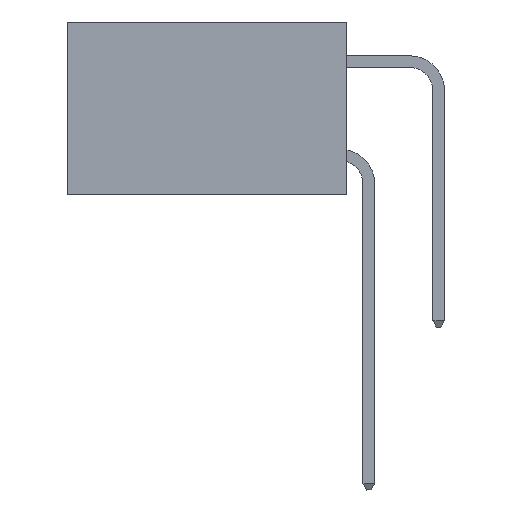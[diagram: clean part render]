
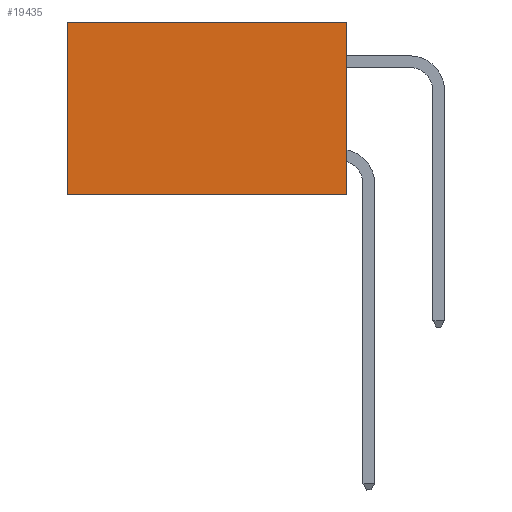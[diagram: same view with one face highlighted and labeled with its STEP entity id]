
A CAD part, left-side view. The second image highlights one B-rep face of the part: STEP entity #19435.
In plain terms, the highlighted planar face has unit normal (-1, 0, 0).
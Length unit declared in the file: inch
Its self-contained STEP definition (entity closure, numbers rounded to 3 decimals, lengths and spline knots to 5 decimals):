
#243 = LINE ( 'NONE', #17175, #26312 ) ;
#957 = AXIS2_PLACEMENT_3D ( 'NONE', #39914, #5919, #27849 ) ;
#1458 = VECTOR ( 'NONE', #9492, 39.37008 ) ;
#1573 = VECTOR ( 'NONE', #36680, 39.37008 ) ;
#1642 = LINE ( 'NONE', #4862, #25771 ) ;
#1814 = EDGE_LOOP ( 'NONE', ( #34650, #26190, #13376, #20717 ) ) ;
#2753 = PLANE ( 'NONE',  #957 ) ;
#4862 = CARTESIAN_POINT ( 'NONE',  ( 0.2875, 0., 0. ) ) ;
#5919 = DIRECTION ( 'NONE',  ( 1., 0., 0. ) ) ;
#8078 = VERTEX_POINT ( 'NONE', #25210 ) ;
#8961 = LINE ( 'NONE', #12013, #1573 ) ;
#9492 = DIRECTION ( 'NONE',  ( 0., 1., 0. ) ) ;
#10827 = LINE ( 'NONE', #34207, #1458 ) ;
#12013 = CARTESIAN_POINT ( 'NONE',  ( 0.2875, 0.6, 0. ) ) ;
#12804 = FACE_OUTER_BOUND ( 'NONE', #1814, .T. ) ;
#13376 = ORIENTED_EDGE ( 'NONE', *, *, #16634, .F. ) ;
#14278 = CARTESIAN_POINT ( 'NONE',  ( 0.2875, 0.6, -0.37 ) ) ;
#16634 = EDGE_CURVE ( 'NONE', #8078, #30290, #243, .T. ) ;
#17175 = CARTESIAN_POINT ( 'NONE',  ( 0.2875, 0., 0. ) ) ;
#17509 = DIRECTION ( 'NONE',  ( 0., 1., 0. ) ) ;
#17941 = VERTEX_POINT ( 'NONE', #14278 ) ;
#19435 = ADVANCED_FACE ( 'NONE', ( #12804 ), #2753, .F. ) ;
#19500 = EDGE_CURVE ( 'NONE', #30290, #17941, #10827, .T. ) ;
#20717 = ORIENTED_EDGE ( 'NONE', *, *, #23862, .T. ) ;
#21933 = CARTESIAN_POINT ( 'NONE',  ( 0.2875, 0., -0.37 ) ) ;
#23862 = EDGE_CURVE ( 'NONE', #8078, #25653, #1642, .T. ) ;
#25210 = CARTESIAN_POINT ( 'NONE',  ( 0.2875, 0., 0. ) ) ;
#25431 = EDGE_CURVE ( 'NONE', #25653, #17941, #8961, .T. ) ;
#25653 = VERTEX_POINT ( 'NONE', #37710 ) ;
#25771 = VECTOR ( 'NONE', #17509, 39.37008 ) ;
#26190 = ORIENTED_EDGE ( 'NONE', *, *, #19500, .F. ) ;
#26312 = VECTOR ( 'NONE', #38700, 39.37008 ) ;
#27849 = DIRECTION ( 'NONE',  ( 0., 0., -1. ) ) ;
#30290 = VERTEX_POINT ( 'NONE', #21933 ) ;
#34207 = CARTESIAN_POINT ( 'NONE',  ( 0.2875, 0., -0.37 ) ) ;
#34650 = ORIENTED_EDGE ( 'NONE', *, *, #25431, .T. ) ;
#36680 = DIRECTION ( 'NONE',  ( 0., 0., -1. ) ) ;
#37710 = CARTESIAN_POINT ( 'NONE',  ( 0.2875, 0.6, 0. ) ) ;
#38700 = DIRECTION ( 'NONE',  ( 0., 0., -1. ) ) ;
#39914 = CARTESIAN_POINT ( 'NONE',  ( 0.2875, 0., 0. ) ) ;
